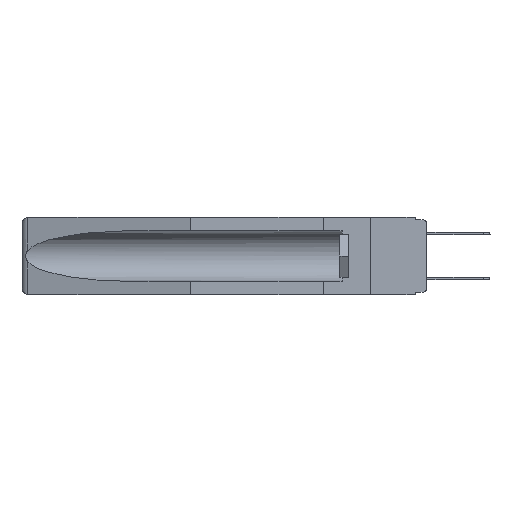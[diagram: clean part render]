
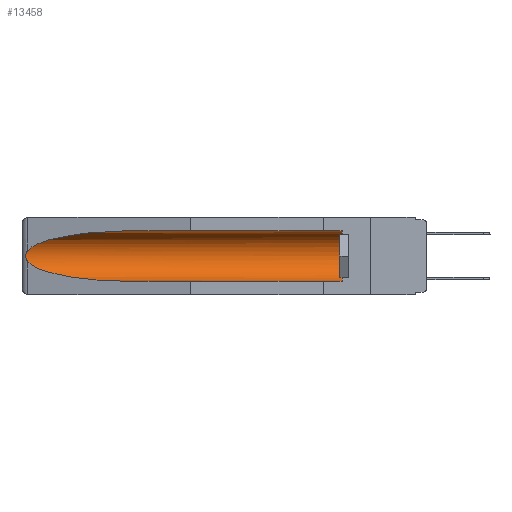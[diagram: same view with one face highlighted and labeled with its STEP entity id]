
A CAD part, left-side view. The second image highlights one B-rep face of the part: STEP entity #13458.
In plain terms, the highlighted cylindrical face has radius 2.857 mm (diameter 5.715 mm), a partial arc.
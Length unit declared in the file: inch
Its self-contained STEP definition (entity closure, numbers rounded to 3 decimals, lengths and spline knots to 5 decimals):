
#245 = CARTESIAN_POINT ( 'NONE',  ( 0.155, 0.126, -0.1715 ) ) ;
#266 = ORIENTED_EDGE ( 'NONE', *, *, #16132, .T. ) ;
#407 = CARTESIAN_POINT ( 'NONE',  ( 0.26597, 1.52961, -0.15275 ) ) ;
#597 = EDGE_LOOP ( 'NONE', ( #8982, #266, #7017, #10838, #4700, #7580 ) ) ;
#707 = CARTESIAN_POINT ( 'NONE',  ( 0.2673, 1.53269, -0.17917 ) ) ;
#1270 = CARTESIAN_POINT ( 'NONE',  ( 0.155, 0.126, -0.284 ) ) ;
#1688 = CARTESIAN_POINT ( 'NONE',  ( 0.155, -0.30754, -0.284 ) ) ;
#1763 = DIRECTION ( 'NONE',  ( 0., -1., 0. ) ) ;
#2218 = CARTESIAN_POINT ( 'NONE',  ( 0.26537, 1.52718, -0.14972 ) ) ;
#2754 = VERTEX_POINT ( 'NONE', #1270 ) ;
#3266 = LINE ( 'NONE', #9425, #16999 ) ;
#3642 =( BOUNDED_CURVE ( )  B_SPLINE_CURVE ( 3, ( #11773, #17890, #4116, #10277 ),
 .UNSPECIFIED., .F., .F. ) 
 B_SPLINE_CURVE_WITH_KNOTS ( ( 4, 4 ),
 ( 0.1948, 1.5708 ),
 .UNSPECIFIED. ) 
 CURVE ( )  GEOMETRIC_REPRESENTATION_ITEM ( )  RATIONAL_B_SPLINE_CURVE ( ( 1., 0.848, 0.848, 1. ) ) 
 REPRESENTATION_ITEM ( '' )  );
#3855 = VECTOR ( 'NONE', #6332, 39.37008 ) ;
#4116 = CARTESIAN_POINT ( 'NONE',  ( 0.21114, 1.30732, -0.284 ) ) ;
#4218 = FACE_OUTER_BOUND ( 'NONE', #597, .T. ) ;
#4700 = ORIENTED_EDGE ( 'NONE', *, *, #7154, .T. ) ;
#4833 = VERTEX_POINT ( 'NONE', #18318 ) ;
#6332 = DIRECTION ( 'NONE',  ( 0., 1., 0. ) ) ;
#6399 = CARTESIAN_POINT ( 'NONE',  ( 0.155, 0.126, -0.059 ) ) ;
#6686 = EDGE_CURVE ( 'NONE', #2754, #19626, #18778, .T. ) ;
#6865 = CARTESIAN_POINT ( 'NONE',  ( 0.26537, 1.52718, -0.19328 ) ) ;
#7017 = ORIENTED_EDGE ( 'NONE', *, *, #10562, .T. ) ;
#7154 = EDGE_CURVE ( 'NONE', #2754, #18670, #12832, .T. ) ;
#7580 = ORIENTED_EDGE ( 'NONE', *, *, #17464, .T. ) ;
#7899 = B_SPLINE_CURVE_WITH_KNOTS ( 'NONE', 3,
 ( #2218, #407, #8281, #11205, #8383, #7979, #707, #14319, #18812, #6865 ),
 .UNSPECIFIED., .F., .F.,
 ( 4, 2, 2, 2, 4 ),
 ( 0., 0.00029, 0.00058, 0.00087, 0.00117 ),
 .UNSPECIFIED. ) ;
#7979 = CARTESIAN_POINT ( 'NONE',  ( 0.2675, 1.53308, -0.17534 ) ) ;
#8281 = CARTESIAN_POINT ( 'NONE',  ( 0.26654, 1.53092, -0.15636 ) ) ;
#8337 = CARTESIAN_POINT ( 'NONE',  ( 0.26537, 1.52718, -0.14972 ) ) ;
#8383 = CARTESIAN_POINT ( 'NONE',  ( 0.2675, 1.53308, -0.16763 ) ) ;
#8982 = ORIENTED_EDGE ( 'NONE', *, *, #15889, .T. ) ;
#9397 = CARTESIAN_POINT ( 'NONE',  ( 0.26537, 1.52718, -0.14972 ) ) ;
#9425 = CARTESIAN_POINT ( 'NONE',  ( 0.155, -0.30754, -0.059 ) ) ;
#9693 = CARTESIAN_POINT ( 'NONE',  ( 0.155, 1.07973, -0.284 ) ) ;
#10277 = CARTESIAN_POINT ( 'NONE',  ( 0.155, 1.07973, -0.284 ) ) ;
#10371 = CARTESIAN_POINT ( 'NONE',  ( 0.155, -0.30754, -0.1715 ) ) ;
#10443 = CARTESIAN_POINT ( 'NONE',  ( 0.25451, 1.48313, -0.09465 ) ) ;
#10562 = EDGE_CURVE ( 'NONE', #14838, #19626, #3642, .T. ) ;
#10838 = ORIENTED_EDGE ( 'NONE', *, *, #6686, .F. ) ;
#11007 = CARTESIAN_POINT ( 'NONE',  ( 0.21114, 1.30732, -0.059 ) ) ;
#11205 = CARTESIAN_POINT ( 'NONE',  ( 0.2673, 1.5327, -0.16383 ) ) ;
#11773 = CARTESIAN_POINT ( 'NONE',  ( 0.26537, 1.52718, -0.19328 ) ) ;
#12832 = CIRCLE ( 'NONE', #14441, 0.1125 ) ;
#13222 = CARTESIAN_POINT ( 'NONE',  ( 0.26537, 1.52718, -0.19328 ) ) ;
#13283 = CYLINDRICAL_SURFACE ( 'NONE', #18835, 0.1125 ) ;
#13458 = ADVANCED_FACE ( 'NONE', ( #4218 ), #13283, .F. ) ;
#13805 = VERTEX_POINT ( 'NONE', #8337 ) ;
#13920 = CARTESIAN_POINT ( 'NONE',  ( 0.155, 1.07973, -0.059 ) ) ;
#14058 = DIRECTION ( 'NONE',  ( 0., 0., 1. ) ) ;
#14319 = CARTESIAN_POINT ( 'NONE',  ( 0.26655, 1.53094, -0.18657 ) ) ;
#14441 = AXIS2_PLACEMENT_3D ( 'NONE', #245, #1763, #14058 ) ;
#14838 = VERTEX_POINT ( 'NONE', #13222 ) ;
#15659 = DIRECTION ( 'NONE',  ( 0., 1., 0. ) ) ;
#15889 = EDGE_CURVE ( 'NONE', #4833, #13805, #16592, .T. ) ;
#16132 = EDGE_CURVE ( 'NONE', #13805, #14838, #7899, .T. ) ;
#16592 =( BOUNDED_CURVE ( )  B_SPLINE_CURVE ( 3, ( #13920, #11007, #10443, #9397 ),
 .UNSPECIFIED., .F., .F. ) 
 B_SPLINE_CURVE_WITH_KNOTS ( ( 4, 4 ),
 ( 4.71239, 6.08839 ),
 .UNSPECIFIED. ) 
 CURVE ( )  GEOMETRIC_REPRESENTATION_ITEM ( )  RATIONAL_B_SPLINE_CURVE ( ( 1., 0.848, 0.848, 1. ) ) 
 REPRESENTATION_ITEM ( '' )  );
#16999 = VECTOR ( 'NONE', #15659, 39.37008 ) ;
#17464 = EDGE_CURVE ( 'NONE', #18670, #4833, #3266, .T. ) ;
#17890 = CARTESIAN_POINT ( 'NONE',  ( 0.25451, 1.48313, -0.24835 ) ) ;
#17891 = DIRECTION ( 'NONE',  ( 0., 0., 1. ) ) ;
#18318 = CARTESIAN_POINT ( 'NONE',  ( 0.155, 1.07973, -0.059 ) ) ;
#18670 = VERTEX_POINT ( 'NONE', #6399 ) ;
#18778 = LINE ( 'NONE', #1688, #3855 ) ;
#18812 = CARTESIAN_POINT ( 'NONE',  ( 0.26597, 1.5296, -0.19026 ) ) ;
#18835 = AXIS2_PLACEMENT_3D ( 'NONE', #10371, #19487, #17891 ) ;
#19487 = DIRECTION ( 'NONE',  ( 0., 1., 0. ) ) ;
#19626 = VERTEX_POINT ( 'NONE', #9693 ) ;
